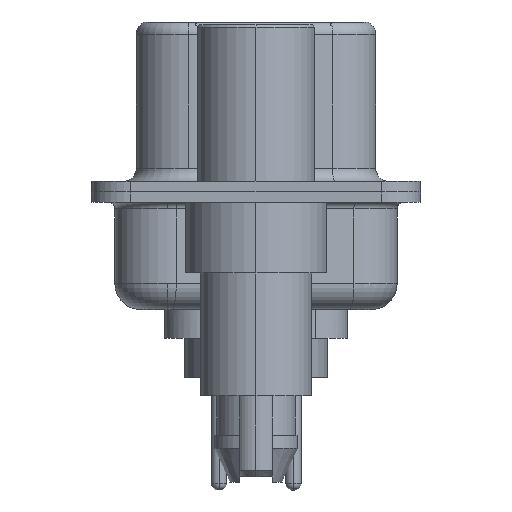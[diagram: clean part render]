
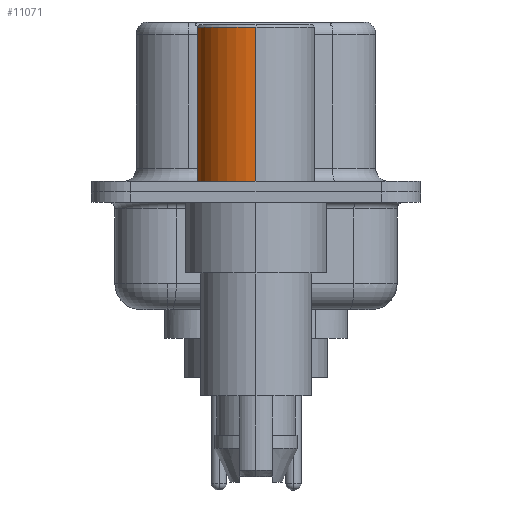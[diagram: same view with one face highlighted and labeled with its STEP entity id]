
A CAD part, left-side view. The second image highlights one B-rep face of the part: STEP entity #11071.
In plain terms, the highlighted cylindrical face has radius 2.25 mm (diameter 4.5 mm), a partial arc.
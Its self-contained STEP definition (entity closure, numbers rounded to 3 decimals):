
#115 = EDGE_CURVE ( 'NONE', #18786, #10801, #15600, .T. ) ;
#2222 = AXIS2_PLACEMENT_3D ( 'NONE', #4229, #22083, #11529 ) ;
#3592 = DIRECTION ( 'NONE',  ( 0., 0., 1. ) ) ;
#4229 = CARTESIAN_POINT ( 'NONE',  ( 0., 0., 0.581 ) ) ;
#4706 = DIRECTION ( 'NONE',  ( 0., 0., 1. ) ) ;
#6442 = CARTESIAN_POINT ( 'NONE',  ( 2.25, 0., 0.581 ) ) ;
#7175 = VECTOR ( 'NONE', #21224, 1000. ) ;
#8342 = VERTEX_POINT ( 'NONE', #16516 ) ;
#8472 = VECTOR ( 'NONE', #17060, 1000. ) ;
#9069 = LINE ( 'NONE', #13514, #8472 ) ;
#9449 = EDGE_CURVE ( 'NONE', #18786, #8342, #12427, .T. ) ;
#9550 = AXIS2_PLACEMENT_3D ( 'NONE', #15455, #4706, #17232 ) ;
#9779 = AXIS2_PLACEMENT_3D ( 'NONE', #14375, #3592, #16184 ) ;
#10337 = CIRCLE ( 'NONE', #9550, 2.25 ) ;
#10801 = VERTEX_POINT ( 'NONE', #10933 ) ;
#10933 = CARTESIAN_POINT ( 'NONE',  ( 2.25, 0., 6.3 ) ) ;
#11071 = ADVANCED_FACE ( 'NONE', ( #20424 ), #18755, .T. ) ;
#11529 = DIRECTION ( 'NONE',  ( 1., 0., 0. ) ) ;
#11794 = ORIENTED_EDGE ( 'NONE', *, *, #115, .F. ) ;
#11964 = ORIENTED_EDGE ( 'NONE', *, *, #18007, .F. ) ;
#12427 = CIRCLE ( 'NONE', #9779, 2.25 ) ;
#13514 = CARTESIAN_POINT ( 'NONE',  ( -2.25, 0., 0.581 ) ) ;
#14375 = CARTESIAN_POINT ( 'NONE',  ( 0., 0., 0.4 ) ) ;
#15455 = CARTESIAN_POINT ( 'NONE',  ( 0., 0., 6.3 ) ) ;
#15600 = LINE ( 'NONE', #6442, #7175 ) ;
#16052 = CARTESIAN_POINT ( 'NONE',  ( 2.25, 0., 0.4 ) ) ;
#16184 = DIRECTION ( 'NONE',  ( 1., 0., 0. ) ) ;
#16516 = CARTESIAN_POINT ( 'NONE',  ( -2.25, 0., 0.4 ) ) ;
#16912 = CARTESIAN_POINT ( 'NONE',  ( -2.25, 0., 6.3 ) ) ;
#17060 = DIRECTION ( 'NONE',  ( 0., 0., 1. ) ) ;
#17232 = DIRECTION ( 'NONE',  ( 1., 0., 0. ) ) ;
#18007 = EDGE_CURVE ( 'NONE', #10801, #22004, #10337, .T. ) ;
#18755 = CYLINDRICAL_SURFACE ( 'NONE', #2222, 2.25 ) ;
#18786 = VERTEX_POINT ( 'NONE', #16052 ) ;
#19779 = ORIENTED_EDGE ( 'NONE', *, *, #21289, .T. ) ;
#20155 = ORIENTED_EDGE ( 'NONE', *, *, #9449, .T. ) ;
#20392 = EDGE_LOOP ( 'NONE', ( #20155, #19779, #11964, #11794 ) ) ;
#20424 = FACE_OUTER_BOUND ( 'NONE', #20392, .T. ) ;
#21224 = DIRECTION ( 'NONE',  ( 0., 0., 1. ) ) ;
#21289 = EDGE_CURVE ( 'NONE', #8342, #22004, #9069, .T. ) ;
#22004 = VERTEX_POINT ( 'NONE', #16912 ) ;
#22083 = DIRECTION ( 'NONE',  ( 0., 0., 1. ) ) ;
